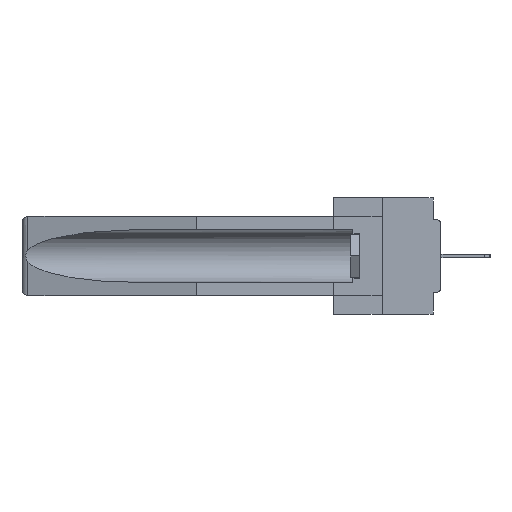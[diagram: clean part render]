
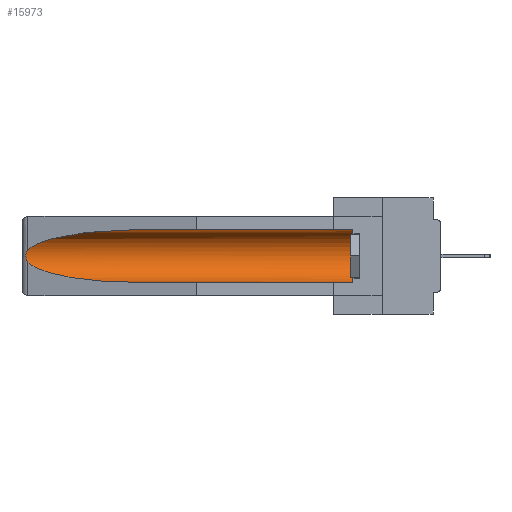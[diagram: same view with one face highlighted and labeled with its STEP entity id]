
A CAD part, left-side view. The second image highlights one B-rep face of the part: STEP entity #15973.
In plain terms, the highlighted cylindrical face has radius 2.857 mm (diameter 5.715 mm), a partial arc.
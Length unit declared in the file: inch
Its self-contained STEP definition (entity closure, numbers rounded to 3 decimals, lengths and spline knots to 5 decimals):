
#305 = VERTEX_POINT ( 'NONE', #12230 ) ;
#557 = VERTEX_POINT ( 'NONE', #24981 ) ;
#1144 = DIRECTION ( 'NONE',  ( 0., 1., 0. ) ) ;
#1191 = ORIENTED_EDGE ( 'NONE', *, *, #27309, .T. ) ;
#1810 = EDGE_CURVE ( 'NONE', #20453, #14891, #18473, .T. ) ;
#3148 = VERTEX_POINT ( 'NONE', #9223 ) ;
#3472 = CARTESIAN_POINT ( 'NONE',  ( 0.26537, 1.52718, -0.14972 ) ) ;
#4098 = CYLINDRICAL_SURFACE ( 'NONE', #24305, 0.1125 ) ;
#4755 = CARTESIAN_POINT ( 'NONE',  ( 0.21114, 1.30732, -0.059 ) ) ;
#4789 = CARTESIAN_POINT ( 'NONE',  ( 0.25451, 1.48313, -0.09465 ) ) ;
#4876 = LINE ( 'NONE', #32526, #17723 ) ;
#5196 = CARTESIAN_POINT ( 'NONE',  ( 0.2673, 1.5327, -0.16383 ) ) ;
#5476 = CARTESIAN_POINT ( 'NONE',  ( 0.155, 0.126, -0.1715 ) ) ;
#5968 = LINE ( 'NONE', #33652, #33909 ) ;
#6494 = AXIS2_PLACEMENT_3D ( 'NONE', #5476, #24536, #8208 ) ;
#7647 = CARTESIAN_POINT ( 'NONE',  ( 0.26537, 1.52718, -0.19328 ) ) ;
#7923 = CARTESIAN_POINT ( 'NONE',  ( 0.2675, 1.53308, -0.17534 ) ) ;
#8208 = DIRECTION ( 'NONE',  ( 0., 0., 1. ) ) ;
#8707 = CARTESIAN_POINT ( 'NONE',  ( 0.26537, 1.52718, -0.14972 ) ) ;
#9223 = CARTESIAN_POINT ( 'NONE',  ( 0.155, 1.07973, -0.284 ) ) ;
#10557 = CARTESIAN_POINT ( 'NONE',  ( 0.26537, 1.52718, -0.14972 ) ) ;
#10681 = CARTESIAN_POINT ( 'NONE',  ( 0.26655, 1.53094, -0.18657 ) ) ;
#11032 = DIRECTION ( 'NONE',  ( 0., 1., 0. ) ) ;
#11263 = ORIENTED_EDGE ( 'NONE', *, *, #24846, .T. ) ;
#11854 = B_SPLINE_CURVE_WITH_KNOTS ( 'NONE', 3,
 ( #10557, #13324, #21564, #5196, #24255, #7923, #26949, #10681, #29657, #13445 ),
 .UNSPECIFIED., .F., .F.,
 ( 4, 2, 2, 2, 4 ),
 ( 0., 0.00029, 0.00058, 0.00087, 0.00117 ),
 .UNSPECIFIED. ) ;
#12230 = CARTESIAN_POINT ( 'NONE',  ( 0.155, 0.126, -0.059 ) ) ;
#13169 = CARTESIAN_POINT ( 'NONE',  ( 0.21114, 1.30732, -0.284 ) ) ;
#13324 = CARTESIAN_POINT ( 'NONE',  ( 0.26597, 1.52961, -0.15275 ) ) ;
#13445 = CARTESIAN_POINT ( 'NONE',  ( 0.26537, 1.52718, -0.19328 ) ) ;
#13643 = DIRECTION ( 'NONE',  ( 0., 1., 0. ) ) ;
#14891 = VERTEX_POINT ( 'NONE', #8707 ) ;
#15973 = ADVANCED_FACE ( 'NONE', ( #33782 ), #4098, .F. ) ;
#16686 =( BOUNDED_CURVE ( )  B_SPLINE_CURVE ( 3, ( #7647, #23969, #13169, #32078 ),
 .UNSPECIFIED., .F., .F. ) 
 B_SPLINE_CURVE_WITH_KNOTS ( ( 4, 4 ),
 ( 0.1948, 1.5708 ),
 .UNSPECIFIED. ) 
 CURVE ( )  GEOMETRIC_REPRESENTATION_ITEM ( )  RATIONAL_B_SPLINE_CURVE ( ( 1., 0.848, 0.848, 1. ) ) 
 REPRESENTATION_ITEM ( '' )  );
#17532 = ORIENTED_EDGE ( 'NONE', *, *, #1810, .T. ) ;
#17723 = VECTOR ( 'NONE', #13643, 39.37008 ) ;
#18295 = CARTESIAN_POINT ( 'NONE',  ( 0.26537, 1.52718, -0.19328 ) ) ;
#18473 =( BOUNDED_CURVE ( )  B_SPLINE_CURVE ( 3, ( #27575, #4755, #4789, #3472 ),
 .UNSPECIFIED., .F., .F. ) 
 B_SPLINE_CURVE_WITH_KNOTS ( ( 4, 4 ),
 ( 4.71239, 6.08839 ),
 .UNSPECIFIED. ) 
 CURVE ( )  GEOMETRIC_REPRESENTATION_ITEM ( )  RATIONAL_B_SPLINE_CURVE ( ( 1., 0.848, 0.848, 1. ) ) 
 REPRESENTATION_ITEM ( '' )  );
#19194 = DIRECTION ( 'NONE',  ( 0., 0., 1. ) ) ;
#20453 = VERTEX_POINT ( 'NONE', #34113 ) ;
#21564 = CARTESIAN_POINT ( 'NONE',  ( 0.26654, 1.53092, -0.15636 ) ) ;
#21765 = ORIENTED_EDGE ( 'NONE', *, *, #31992, .T. ) ;
#23450 = ORIENTED_EDGE ( 'NONE', *, *, #23659, .T. ) ;
#23480 = EDGE_LOOP ( 'NONE', ( #17532, #23450, #21765, #29964, #11263, #1191 ) ) ;
#23659 = EDGE_CURVE ( 'NONE', #14891, #34044, #11854, .T. ) ;
#23969 = CARTESIAN_POINT ( 'NONE',  ( 0.25451, 1.48313, -0.24835 ) ) ;
#24255 = CARTESIAN_POINT ( 'NONE',  ( 0.2675, 1.53308, -0.16763 ) ) ;
#24305 = AXIS2_PLACEMENT_3D ( 'NONE', #27302, #11032, #19194 ) ;
#24536 = DIRECTION ( 'NONE',  ( 0., -1., 0. ) ) ;
#24846 = EDGE_CURVE ( 'NONE', #557, #305, #32047, .T. ) ;
#24981 = CARTESIAN_POINT ( 'NONE',  ( 0.155, 0.126, -0.284 ) ) ;
#26949 = CARTESIAN_POINT ( 'NONE',  ( 0.2673, 1.53269, -0.17917 ) ) ;
#27302 = CARTESIAN_POINT ( 'NONE',  ( 0.155, -0.30754, -0.1715 ) ) ;
#27309 = EDGE_CURVE ( 'NONE', #305, #20453, #5968, .T. ) ;
#27575 = CARTESIAN_POINT ( 'NONE',  ( 0.155, 1.07973, -0.059 ) ) ;
#29657 = CARTESIAN_POINT ( 'NONE',  ( 0.26597, 1.5296, -0.19026 ) ) ;
#29964 = ORIENTED_EDGE ( 'NONE', *, *, #32148, .F. ) ;
#31992 = EDGE_CURVE ( 'NONE', #34044, #3148, #16686, .T. ) ;
#32047 = CIRCLE ( 'NONE', #6494, 0.1125 ) ;
#32078 = CARTESIAN_POINT ( 'NONE',  ( 0.155, 1.07973, -0.284 ) ) ;
#32148 = EDGE_CURVE ( 'NONE', #557, #3148, #4876, .T. ) ;
#32526 = CARTESIAN_POINT ( 'NONE',  ( 0.155, -0.30754, -0.284 ) ) ;
#33652 = CARTESIAN_POINT ( 'NONE',  ( 0.155, -0.30754, -0.059 ) ) ;
#33782 = FACE_OUTER_BOUND ( 'NONE', #23480, .T. ) ;
#33909 = VECTOR ( 'NONE', #1144, 39.37008 ) ;
#34044 = VERTEX_POINT ( 'NONE', #18295 ) ;
#34113 = CARTESIAN_POINT ( 'NONE',  ( 0.155, 1.07973, -0.059 ) ) ;
